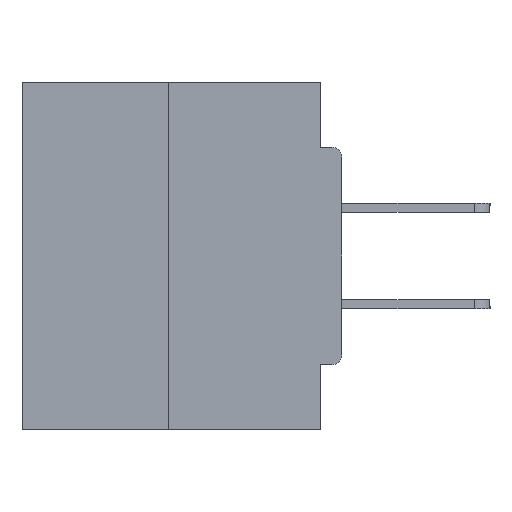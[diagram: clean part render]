
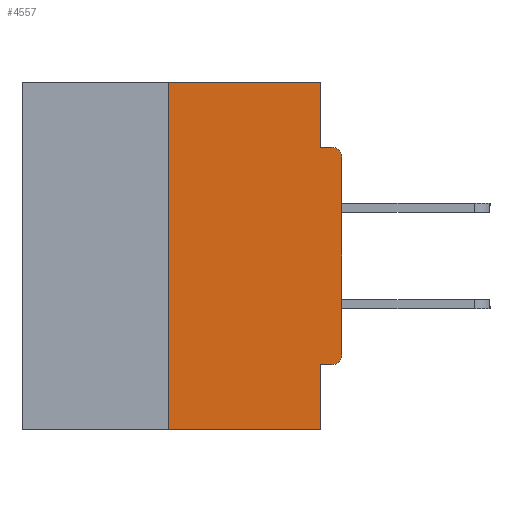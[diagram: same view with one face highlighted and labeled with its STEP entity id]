
A CAD part, left-side view. The second image highlights one B-rep face of the part: STEP entity #4557.
In plain terms, the highlighted planar face has unit normal (-1, 0, 0).
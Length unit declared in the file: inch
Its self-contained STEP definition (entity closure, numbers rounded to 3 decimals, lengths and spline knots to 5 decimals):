
#146 = CARTESIAN_POINT ( 'NONE',  ( 0., 0., -0.3915 ) ) ;
#206 = CARTESIAN_POINT ( 'NONE',  ( 0., 0.015, -0.3915 ) ) ;
#267 = VERTEX_POINT ( 'NONE', #27310 ) ;
#646 = EDGE_CURVE ( 'NONE', #42441, #267, #28329, .T. ) ;
#673 = CARTESIAN_POINT ( 'NONE',  ( 0., 0.031, -0.4065 ) ) ;
#774 = CARTESIAN_POINT ( 'NONE',  ( 0., 0.25, 0. ) ) ;
#1204 = EDGE_CURVE ( 'NONE', #38755, #11423, #9821, .T. ) ;
#1219 = ORIENTED_EDGE ( 'NONE', *, *, #2165, .T. ) ;
#2165 = EDGE_CURVE ( 'NONE', #13365, #28658, #35220, .T. ) ;
#2408 = DIRECTION ( 'NONE',  ( 0., 0., -1. ) ) ;
#3237 = CARTESIAN_POINT ( 'NONE',  ( 0., 0., -0.0935 ) ) ;
#3317 = EDGE_LOOP ( 'NONE', ( #9959, #28636, #29716, #23082, #22959, #9310, #9336, #1219, #29713, #4705 ) ) ;
#3457 = CARTESIAN_POINT ( 'NONE',  ( 0., 0.46, 0. ) ) ;
#3557 = CARTESIAN_POINT ( 'NONE',  ( 0., 0.25, -0.5 ) ) ;
#4059 = DIRECTION ( 'NONE',  ( -1., 0., 0. ) ) ;
#4557 = ADVANCED_FACE ( 'NONE', ( #22845 ), #25351, .F. ) ;
#4705 = ORIENTED_EDGE ( 'NONE', *, *, #38706, .F. ) ;
#4819 = EDGE_CURVE ( 'NONE', #41539, #267, #12140, .T. ) ;
#6837 = DIRECTION ( 'NONE',  ( 0., 0., -1. ) ) ;
#8360 = DIRECTION ( 'NONE',  ( 0., 0., -1. ) ) ;
#8450 = CARTESIAN_POINT ( 'NONE',  ( 0., 0.46, 0. ) ) ;
#8649 = CARTESIAN_POINT ( 'NONE',  ( 0., 0.015, -0.1085 ) ) ;
#9310 = ORIENTED_EDGE ( 'NONE', *, *, #34778, .T. ) ;
#9336 = ORIENTED_EDGE ( 'NONE', *, *, #10160, .T. ) ;
#9455 = LINE ( 'NONE', #3237, #14197 ) ;
#9821 = LINE ( 'NONE', #3457, #16150 ) ;
#9959 = ORIENTED_EDGE ( 'NONE', *, *, #1204, .F. ) ;
#10160 = EDGE_CURVE ( 'NONE', #36495, #13365, #21751, .T. ) ;
#10496 = DIRECTION ( 'NONE',  ( 0., 0., 1. ) ) ;
#11423 = VERTEX_POINT ( 'NONE', #20508 ) ;
#12140 = LINE ( 'NONE', #12201, #28114 ) ;
#12150 = VECTOR ( 'NONE', #37346, 39.37008 ) ;
#12201 = CARTESIAN_POINT ( 'NONE',  ( 0., 0.031, -0.5 ) ) ;
#13365 = VERTEX_POINT ( 'NONE', #32753 ) ;
#13407 = CARTESIAN_POINT ( 'NONE',  ( 0., 0.031, 0. ) ) ;
#13618 = CARTESIAN_POINT ( 'NONE',  ( 0., 0., 0. ) ) ;
#14197 = VECTOR ( 'NONE', #16512, 39.37008 ) ;
#14354 = DIRECTION ( 'NONE',  ( 0., -1., 0. ) ) ;
#14786 = EDGE_CURVE ( 'NONE', #35694, #28658, #9455, .T. ) ;
#14929 = VECTOR ( 'NONE', #10496, 39.37008 ) ;
#16150 = VECTOR ( 'NONE', #14354, 39.37008 ) ;
#16512 = DIRECTION ( 'NONE',  ( 0., -1., 0. ) ) ;
#16970 = AXIS2_PLACEMENT_3D ( 'NONE', #206, #4059, #6837 ) ;
#17628 = DIRECTION ( 'NONE',  ( 0., 1., 0. ) ) ;
#20117 = DIRECTION ( 'NONE',  ( 0., 0., -1. ) ) ;
#20508 = CARTESIAN_POINT ( 'NONE',  ( 0., 0.031, 0. ) ) ;
#21751 = LINE ( 'NONE', #13618, #12150 ) ;
#21888 = EDGE_CURVE ( 'NONE', #38363, #41539, #43632, .T. ) ;
#22845 = FACE_OUTER_BOUND ( 'NONE', #3317, .T. ) ;
#22959 = ORIENTED_EDGE ( 'NONE', *, *, #21888, .F. ) ;
#23082 = ORIENTED_EDGE ( 'NONE', *, *, #4819, .F. ) ;
#23430 = LINE ( 'NONE', #774, #14929 ) ;
#24618 = VECTOR ( 'NONE', #17628, 39.37008 ) ;
#25055 = AXIS2_PLACEMENT_3D ( 'NONE', #8450, #32163, #2408 ) ;
#25351 = PLANE ( 'NONE',  #25055 ) ;
#26515 = CARTESIAN_POINT ( 'NONE',  ( 0., 0.46, -0.5 ) ) ;
#27246 = CARTESIAN_POINT ( 'NONE',  ( 0., 0.25, 0. ) ) ;
#27310 = CARTESIAN_POINT ( 'NONE',  ( 0., 0.031, -0.5 ) ) ;
#27806 = VECTOR ( 'NONE', #39525, 39.37008 ) ;
#28114 = VECTOR ( 'NONE', #38780, 39.37008 ) ;
#28181 = CARTESIAN_POINT ( 'NONE',  ( 0., 0.015, -0.0935 ) ) ;
#28329 = LINE ( 'NONE', #26515, #27806 ) ;
#28636 = ORIENTED_EDGE ( 'NONE', *, *, #37156, .F. ) ;
#28658 = VERTEX_POINT ( 'NONE', #28181 ) ;
#29283 = CARTESIAN_POINT ( 'NONE',  ( 0., 0.031, -0.0935 ) ) ;
#29713 = ORIENTED_EDGE ( 'NONE', *, *, #14786, .F. ) ;
#29716 = ORIENTED_EDGE ( 'NONE', *, *, #646, .T. ) ;
#31785 = AXIS2_PLACEMENT_3D ( 'NONE', #8649, #42257, #8360 ) ;
#32163 = DIRECTION ( 'NONE',  ( 1., 0., 0. ) ) ;
#32753 = CARTESIAN_POINT ( 'NONE',  ( 0., 0., -0.1085 ) ) ;
#34778 = EDGE_CURVE ( 'NONE', #38363, #36495, #42697, .T. ) ;
#35220 = CIRCLE ( 'NONE', #31785, 0.015 ) ;
#35694 = VERTEX_POINT ( 'NONE', #29283 ) ;
#36495 = VERTEX_POINT ( 'NONE', #146 ) ;
#37156 = EDGE_CURVE ( 'NONE', #42441, #38755, #23430, .T. ) ;
#37346 = DIRECTION ( 'NONE',  ( 0., 0., 1. ) ) ;
#38363 = VERTEX_POINT ( 'NONE', #41034 ) ;
#38706 = EDGE_CURVE ( 'NONE', #11423, #35694, #42260, .T. ) ;
#38755 = VERTEX_POINT ( 'NONE', #27246 ) ;
#38780 = DIRECTION ( 'NONE',  ( 0., 0., -1. ) ) ;
#39525 = DIRECTION ( 'NONE',  ( 0., -1., 0. ) ) ;
#41034 = CARTESIAN_POINT ( 'NONE',  ( 0., 0.015, -0.4065 ) ) ;
#41194 = VECTOR ( 'NONE', #20117, 39.37008 ) ;
#41539 = VERTEX_POINT ( 'NONE', #673 ) ;
#41916 = CARTESIAN_POINT ( 'NONE',  ( 0., 0., -0.4065 ) ) ;
#42257 = DIRECTION ( 'NONE',  ( -1., 0., 0. ) ) ;
#42260 = LINE ( 'NONE', #13407, #41194 ) ;
#42441 = VERTEX_POINT ( 'NONE', #3557 ) ;
#42697 = CIRCLE ( 'NONE', #16970, 0.015 ) ;
#43632 = LINE ( 'NONE', #41916, #24618 ) ;
